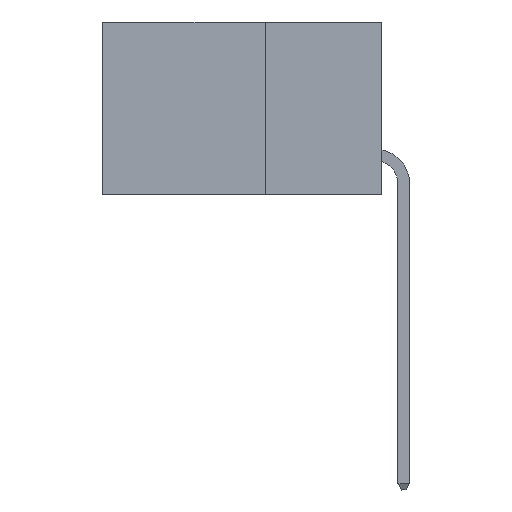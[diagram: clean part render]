
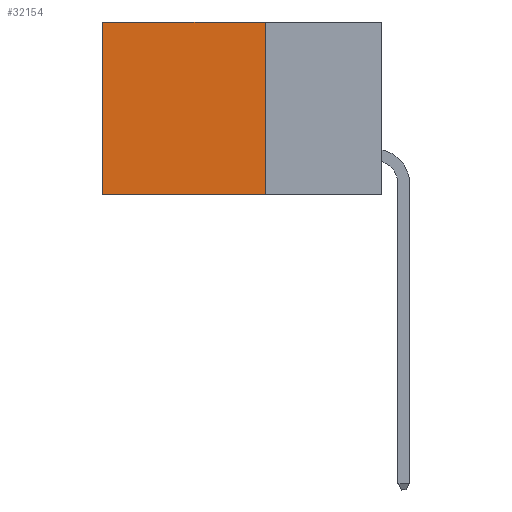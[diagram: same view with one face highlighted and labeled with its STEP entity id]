
A CAD part, left-side view. The second image highlights one B-rep face of the part: STEP entity #32154.
In plain terms, the highlighted planar face has unit normal (-1, 0, 0).
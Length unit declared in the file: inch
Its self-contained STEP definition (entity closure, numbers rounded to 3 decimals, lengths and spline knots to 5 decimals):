
#1225 = LINE ( 'NONE', #23916, #27959 ) ;
#1391 = DIRECTION ( 'NONE',  ( 1., 0., 0. ) ) ;
#3288 = VERTEX_POINT ( 'NONE', #13296 ) ;
#5445 = EDGE_CURVE ( 'NONE', #29986, #19427, #20412, .T. ) ;
#5710 = DIRECTION ( 'NONE',  ( 0., 1., 0. ) ) ;
#6635 = VECTOR ( 'NONE', #9745, 39.37008 ) ;
#7603 = PLANE ( 'NONE',  #8633 ) ;
#7913 = CARTESIAN_POINT ( 'NONE',  ( 0.2875, 0.25, 0. ) ) ;
#8633 = AXIS2_PLACEMENT_3D ( 'NONE', #10281, #1391, #29473 ) ;
#8877 = ORIENTED_EDGE ( 'NONE', *, *, #22922, .T. ) ;
#9745 = DIRECTION ( 'NONE',  ( 0., 0., -1. ) ) ;
#9793 = CARTESIAN_POINT ( 'NONE',  ( 0.2875, 0.25, -0.37 ) ) ;
#9853 = EDGE_CURVE ( 'NONE', #19427, #3288, #16376, .T. ) ;
#10009 = FACE_OUTER_BOUND ( 'NONE', #11721, .T. ) ;
#10281 = CARTESIAN_POINT ( 'NONE',  ( 0.2875, 0.25, 0. ) ) ;
#11089 = CARTESIAN_POINT ( 'NONE',  ( 0.2875, 0.6, 0. ) ) ;
#11721 = EDGE_LOOP ( 'NONE', ( #8877, #22708, #22797, #11932 ) ) ;
#11932 = ORIENTED_EDGE ( 'NONE', *, *, #28126, .T. ) ;
#11946 = DIRECTION ( 'NONE',  ( 0., 0., -1. ) ) ;
#13296 = CARTESIAN_POINT ( 'NONE',  ( 0.2875, 0.6, -0.37 ) ) ;
#16376 = LINE ( 'NONE', #9793, #27347 ) ;
#17598 = DIRECTION ( 'NONE',  ( 0., 1., 0. ) ) ;
#19427 = VERTEX_POINT ( 'NONE', #28934 ) ;
#19604 = CARTESIAN_POINT ( 'NONE',  ( 0.2875, 0.25, 0. ) ) ;
#20412 = LINE ( 'NONE', #7913, #6635 ) ;
#22708 = ORIENTED_EDGE ( 'NONE', *, *, #9853, .F. ) ;
#22797 = ORIENTED_EDGE ( 'NONE', *, *, #5445, .F. ) ;
#22922 = EDGE_CURVE ( 'NONE', #29778, #3288, #30386, .T. ) ;
#23916 = CARTESIAN_POINT ( 'NONE',  ( 0.2875, 0.25, 0. ) ) ;
#26783 = CARTESIAN_POINT ( 'NONE',  ( 0.2875, 0.6, 0. ) ) ;
#27347 = VECTOR ( 'NONE', #17598, 39.37008 ) ;
#27531 = VECTOR ( 'NONE', #11946, 39.37008 ) ;
#27959 = VECTOR ( 'NONE', #5710, 39.37008 ) ;
#28126 = EDGE_CURVE ( 'NONE', #29986, #29778, #1225, .T. ) ;
#28934 = CARTESIAN_POINT ( 'NONE',  ( 0.2875, 0.25, -0.37 ) ) ;
#29473 = DIRECTION ( 'NONE',  ( 0., 0., -1. ) ) ;
#29778 = VERTEX_POINT ( 'NONE', #11089 ) ;
#29986 = VERTEX_POINT ( 'NONE', #19604 ) ;
#30386 = LINE ( 'NONE', #26783, #27531 ) ;
#32154 = ADVANCED_FACE ( 'NONE', ( #10009 ), #7603, .F. ) ;
